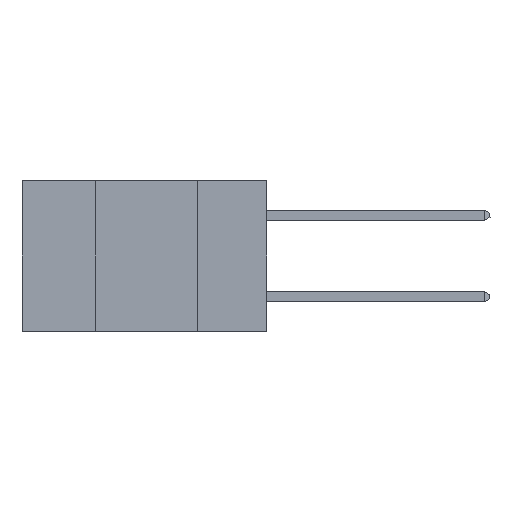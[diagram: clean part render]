
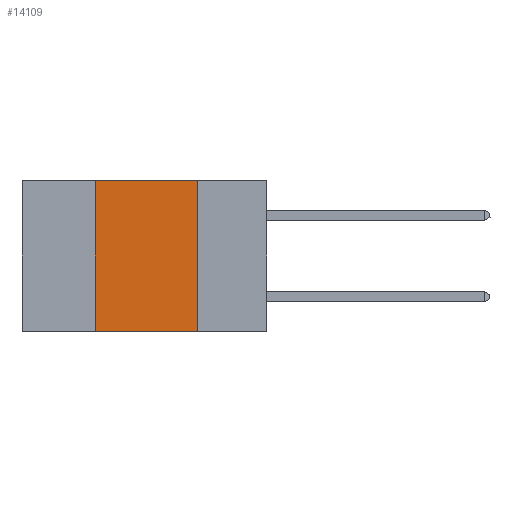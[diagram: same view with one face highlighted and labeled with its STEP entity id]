
A CAD part, left-side view. The second image highlights one B-rep face of the part: STEP entity #14109.
In plain terms, the highlighted planar face has unit normal (-1, 0, 0).
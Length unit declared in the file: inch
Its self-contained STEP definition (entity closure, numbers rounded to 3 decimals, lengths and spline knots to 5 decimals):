
#1471 = VECTOR ( 'NONE', #15433, 39.37008 ) ;
#2294 = VECTOR ( 'NONE', #6140, 39.37008 ) ;
#2447 = CARTESIAN_POINT ( 'NONE',  ( 0., 0.6, 0. ) ) ;
#2563 = ORIENTED_EDGE ( 'NONE', *, *, #10217, .F. ) ;
#2611 = CARTESIAN_POINT ( 'NONE',  ( 0., 0.17, -0.37 ) ) ;
#3306 = VECTOR ( 'NONE', #12727, 39.37008 ) ;
#3808 = CARTESIAN_POINT ( 'NONE',  ( 0., 0.6, -0.37 ) ) ;
#3905 = LINE ( 'NONE', #8929, #10993 ) ;
#4362 = VERTEX_POINT ( 'NONE', #2611 ) ;
#5141 = PLANE ( 'NONE',  #16408 ) ;
#6140 = DIRECTION ( 'NONE',  ( 0., -1., 0. ) ) ;
#6580 = CARTESIAN_POINT ( 'NONE',  ( 0., 0.42, 0. ) ) ;
#6775 = EDGE_CURVE ( 'NONE', #9139, #9968, #8002, .T. ) ;
#6983 = EDGE_CURVE ( 'NONE', #9139, #4362, #16599, .T. ) ;
#7568 = DIRECTION ( 'NONE',  ( 0., 0., -1. ) ) ;
#7727 = LINE ( 'NONE', #2447, #3306 ) ;
#8002 = LINE ( 'NONE', #6580, #1471 ) ;
#8053 = ORIENTED_EDGE ( 'NONE', *, *, #6775, .F. ) ;
#8929 = CARTESIAN_POINT ( 'NONE',  ( 0., 0.17, 0. ) ) ;
#9139 = VERTEX_POINT ( 'NONE', #14563 ) ;
#9504 = ORIENTED_EDGE ( 'NONE', *, *, #10731, .F. ) ;
#9968 = VERTEX_POINT ( 'NONE', #10350 ) ;
#10048 = DIRECTION ( 'NONE',  ( 1., 0., 0. ) ) ;
#10209 = FACE_OUTER_BOUND ( 'NONE', #10348, .T. ) ;
#10217 = EDGE_CURVE ( 'NONE', #15486, #4362, #3905, .T. ) ;
#10348 = EDGE_LOOP ( 'NONE', ( #2563, #9504, #8053, #13270 ) ) ;
#10350 = CARTESIAN_POINT ( 'NONE',  ( 0., 0.42, 0. ) ) ;
#10731 = EDGE_CURVE ( 'NONE', #9968, #15486, #7727, .T. ) ;
#10993 = VECTOR ( 'NONE', #11380, 39.37008 ) ;
#11380 = DIRECTION ( 'NONE',  ( 0., 0., -1. ) ) ;
#12727 = DIRECTION ( 'NONE',  ( 0., -1., 0. ) ) ;
#13270 = ORIENTED_EDGE ( 'NONE', *, *, #6983, .T. ) ;
#13824 = CARTESIAN_POINT ( 'NONE',  ( 0., 0.6, 0. ) ) ;
#14109 = ADVANCED_FACE ( 'NONE', ( #10209 ), #5141, .F. ) ;
#14396 = CARTESIAN_POINT ( 'NONE',  ( 0., 0.17, 0. ) ) ;
#14563 = CARTESIAN_POINT ( 'NONE',  ( 0., 0.42, -0.37 ) ) ;
#15433 = DIRECTION ( 'NONE',  ( 0., 0., 1. ) ) ;
#15486 = VERTEX_POINT ( 'NONE', #14396 ) ;
#16408 = AXIS2_PLACEMENT_3D ( 'NONE', #13824, #10048, #7568 ) ;
#16599 = LINE ( 'NONE', #3808, #2294 ) ;
